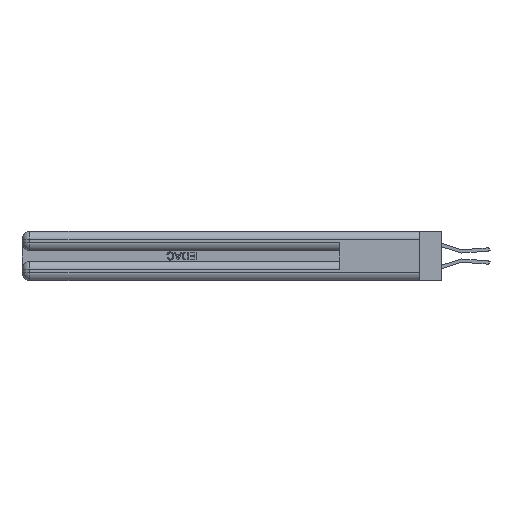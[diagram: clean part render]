
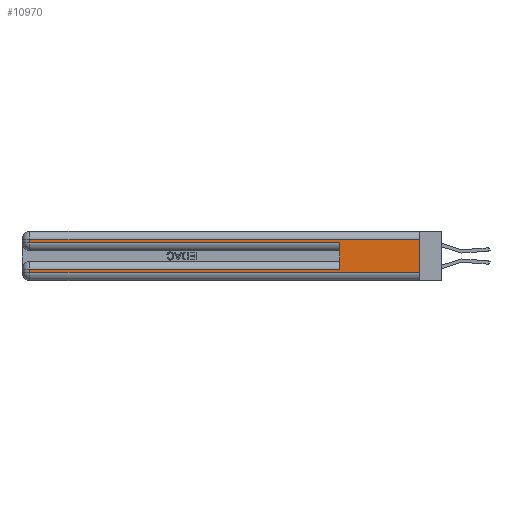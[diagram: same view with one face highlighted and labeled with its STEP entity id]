
A CAD part, left-side view. The second image highlights one B-rep face of the part: STEP entity #10970.
In plain terms, the highlighted planar face has unit normal (-1, 0, 0).
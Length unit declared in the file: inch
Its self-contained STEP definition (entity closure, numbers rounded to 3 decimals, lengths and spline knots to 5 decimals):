
#594 = DIRECTION ( 'NONE',  ( 0., 0., 1. ) ) ;
#755 = VERTEX_POINT ( 'NONE', #32527 ) ;
#867 = CARTESIAN_POINT ( 'NONE',  ( 0., 0.6, 0.145 ) ) ;
#1088 = PLANE ( 'NONE',  #37337 ) ;
#1196 = DIRECTION ( 'NONE',  ( 0., 0., -1. ) ) ;
#1669 = VERTEX_POINT ( 'NONE', #30081 ) ;
#2265 = EDGE_CURVE ( 'NONE', #10382, #32856, #12992, .T. ) ;
#2660 = EDGE_CURVE ( 'NONE', #1669, #36854, #18444, .T. ) ;
#2800 = VECTOR ( 'NONE', #34976, 39.37008 ) ;
#3094 = VECTOR ( 'NONE', #25934, 39.37008 ) ;
#3127 = ORIENTED_EDGE ( 'NONE', *, *, #20509, .T. ) ;
#3366 = LINE ( 'NONE', #36679, #2800 ) ;
#5367 = CARTESIAN_POINT ( 'NONE',  ( 0., 0., 0.06 ) ) ;
#5508 = EDGE_CURVE ( 'NONE', #6826, #36854, #3366, .T. ) ;
#5586 = CARTESIAN_POINT ( 'NONE',  ( 0., 0., 0.37 ) ) ;
#6217 = ORIENTED_EDGE ( 'NONE', *, *, #41424, .T. ) ;
#6379 = VECTOR ( 'NONE', #23862, 39.37008 ) ;
#6511 = EDGE_CURVE ( 'NONE', #29015, #26497, #13115, .T. ) ;
#6826 = VERTEX_POINT ( 'NONE', #34781 ) ;
#8300 = VECTOR ( 'NONE', #30845, 39.37008 ) ;
#8629 = CARTESIAN_POINT ( 'NONE',  ( 0., 2.94, 0.37 ) ) ;
#8642 = DIRECTION ( 'NONE',  ( 0., 1., 0. ) ) ;
#9088 = ORIENTED_EDGE ( 'NONE', *, *, #2265, .F. ) ;
#9124 = VECTOR ( 'NONE', #594, 39.37008 ) ;
#10286 = EDGE_CURVE ( 'NONE', #755, #6826, #33753, .T. ) ;
#10382 = VERTEX_POINT ( 'NONE', #30842 ) ;
#10422 = LINE ( 'NONE', #30176, #29729 ) ;
#10970 = ADVANCED_FACE ( 'NONE', ( #23259 ), #1088, .F. ) ;
#12199 = DIRECTION ( 'NONE',  ( 0., 0., -1. ) ) ;
#12589 = VECTOR ( 'NONE', #1196, 39.37008 ) ;
#12738 = LINE ( 'NONE', #27306, #8300 ) ;
#12992 = LINE ( 'NONE', #37732, #6379 ) ;
#13115 = LINE ( 'NONE', #8629, #12589 ) ;
#13981 = ORIENTED_EDGE ( 'NONE', *, *, #10286, .T. ) ;
#18444 = LINE ( 'NONE', #867, #9124 ) ;
#18668 = CARTESIAN_POINT ( 'NONE',  ( 0., 2.94, 0.37 ) ) ;
#18843 = ORIENTED_EDGE ( 'NONE', *, *, #6511, .T. ) ;
#19300 = ORIENTED_EDGE ( 'NONE', *, *, #2660, .F. ) ;
#20509 = EDGE_CURVE ( 'NONE', #26497, #32856, #12738, .T. ) ;
#22080 = DIRECTION ( 'NONE',  ( 0., 0., -1. ) ) ;
#22574 = CARTESIAN_POINT ( 'NONE',  ( 0., 0., 0.085 ) ) ;
#23259 = FACE_OUTER_BOUND ( 'NONE', #45501, .T. ) ;
#23862 = DIRECTION ( 'NONE',  ( 0., 0., -1. ) ) ;
#23980 = ORIENTED_EDGE ( 'NONE', *, *, #5508, .T. ) ;
#25934 = DIRECTION ( 'NONE',  ( 0., 1., 0. ) ) ;
#26371 = DIRECTION ( 'NONE',  ( 1., 0., 0. ) ) ;
#26497 = VERTEX_POINT ( 'NONE', #42743 ) ;
#26843 = CARTESIAN_POINT ( 'NONE',  ( 0., 2.94, 0.085 ) ) ;
#27306 = CARTESIAN_POINT ( 'NONE',  ( 0., 0., 0.06 ) ) ;
#29015 = VERTEX_POINT ( 'NONE', #26843 ) ;
#29729 = VECTOR ( 'NONE', #8642, 39.37008 ) ;
#30081 = CARTESIAN_POINT ( 'NONE',  ( 0., 0.6, 0.085 ) ) ;
#30176 = CARTESIAN_POINT ( 'NONE',  ( 0., 0., 0.31 ) ) ;
#30842 = CARTESIAN_POINT ( 'NONE',  ( 0., 0., 0.31 ) ) ;
#30845 = DIRECTION ( 'NONE',  ( 0., -1., 0. ) ) ;
#32527 = CARTESIAN_POINT ( 'NONE',  ( 0., 2.94, 0.31 ) ) ;
#32856 = VERTEX_POINT ( 'NONE', #5367 ) ;
#33753 = LINE ( 'NONE', #18668, #45309 ) ;
#34781 = CARTESIAN_POINT ( 'NONE',  ( 0., 2.94, 0.285 ) ) ;
#34976 = DIRECTION ( 'NONE',  ( 0., -1., 0. ) ) ;
#36269 = ORIENTED_EDGE ( 'NONE', *, *, #43118, .T. ) ;
#36679 = CARTESIAN_POINT ( 'NONE',  ( 0., 0., 0.285 ) ) ;
#36686 = LINE ( 'NONE', #22574, #3094 ) ;
#36854 = VERTEX_POINT ( 'NONE', #37157 ) ;
#37157 = CARTESIAN_POINT ( 'NONE',  ( 0., 0.6, 0.285 ) ) ;
#37337 = AXIS2_PLACEMENT_3D ( 'NONE', #5586, #26371, #12199 ) ;
#37732 = CARTESIAN_POINT ( 'NONE',  ( 0., 0., 0.37 ) ) ;
#41424 = EDGE_CURVE ( 'NONE', #10382, #755, #10422, .T. ) ;
#42743 = CARTESIAN_POINT ( 'NONE',  ( 0., 2.94, 0.06 ) ) ;
#43118 = EDGE_CURVE ( 'NONE', #1669, #29015, #36686, .T. ) ;
#45309 = VECTOR ( 'NONE', #22080, 39.37008 ) ;
#45501 = EDGE_LOOP ( 'NONE', ( #9088, #6217, #13981, #23980, #19300, #36269, #18843, #3127 ) ) ;
